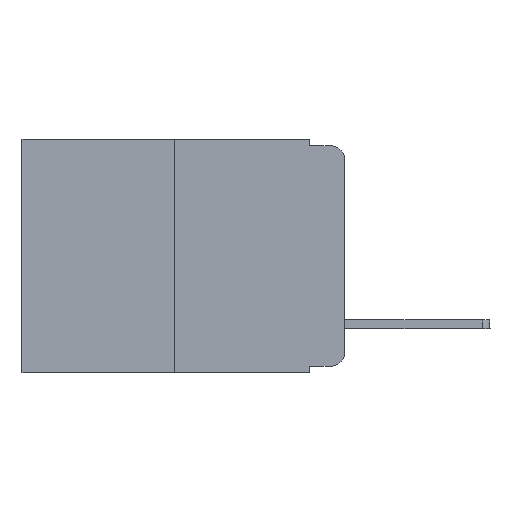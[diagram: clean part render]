
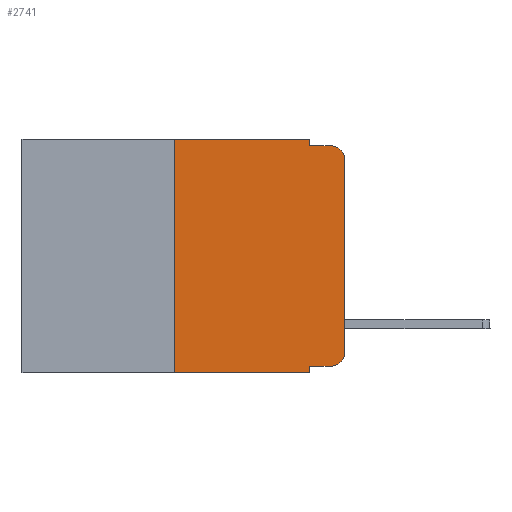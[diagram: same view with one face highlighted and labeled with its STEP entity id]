
A CAD part, left-side view. The second image highlights one B-rep face of the part: STEP entity #2741.
In plain terms, the highlighted planar face has unit normal (-1, 0, 0).
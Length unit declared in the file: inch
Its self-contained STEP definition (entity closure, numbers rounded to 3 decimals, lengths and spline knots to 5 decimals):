
#124 = VECTOR ( 'NONE', #4644, 39.37008 ) ;
#211 = EDGE_CURVE ( 'NONE', #13435, #8046, #12303, .T. ) ;
#518 = EDGE_CURVE ( 'NONE', #3727, #5119, #7516, .T. ) ;
#966 = ORIENTED_EDGE ( 'NONE', *, *, #2145, .T. ) ;
#1111 = VECTOR ( 'NONE', #12831, 39.37008 ) ;
#1455 = VERTEX_POINT ( 'NONE', #7439 ) ;
#1536 = CARTESIAN_POINT ( 'NONE',  ( 0., 0.473, 0. ) ) ;
#1609 = ORIENTED_EDGE ( 'NONE', *, *, #13899, .T. ) ;
#1706 = LINE ( 'NONE', #11536, #1111 ) ;
#1962 = CARTESIAN_POINT ( 'NONE',  ( 0., 0.25, -0.343 ) ) ;
#2133 = CARTESIAN_POINT ( 'NONE',  ( 0., 0.02, -0.01 ) ) ;
#2145 = EDGE_CURVE ( 'NONE', #16612, #15580, #2423, .T. ) ;
#2423 = LINE ( 'NONE', #12483, #6634 ) ;
#2518 = AXIS2_PLACEMENT_3D ( 'NONE', #11766, #15399, #14137 ) ;
#2538 = EDGE_CURVE ( 'NONE', #15580, #13642, #10623, .T. ) ;
#2741 = ADVANCED_FACE ( 'NONE', ( #5210 ), #16152, .F. ) ;
#3237 = DIRECTION ( 'NONE',  ( -1., 0., 0. ) ) ;
#3691 = CARTESIAN_POINT ( 'NONE',  ( 0., 0.051, 0. ) ) ;
#3693 = DIRECTION ( 'NONE',  ( 0., 0., -1. ) ) ;
#3702 = VECTOR ( 'NONE', #6491, 39.37008 ) ;
#3727 = VERTEX_POINT ( 'NONE', #7046 ) ;
#4431 = ORIENTED_EDGE ( 'NONE', *, *, #518, .F. ) ;
#4644 = DIRECTION ( 'NONE',  ( 0., -1., 0. ) ) ;
#4692 = VECTOR ( 'NONE', #10148, 39.37008 ) ;
#5088 = EDGE_CURVE ( 'NONE', #13435, #1455, #7378, .T. ) ;
#5119 = VERTEX_POINT ( 'NONE', #8451 ) ;
#5207 = CARTESIAN_POINT ( 'NONE',  ( 0., 0.051, -0.333 ) ) ;
#5210 = FACE_OUTER_BOUND ( 'NONE', #14205, .T. ) ;
#5628 = CARTESIAN_POINT ( 'NONE',  ( 0., 0.25, 0. ) ) ;
#5692 = LINE ( 'NONE', #1536, #3702 ) ;
#5862 = LINE ( 'NONE', #7553, #15664 ) ;
#6204 = DIRECTION ( 'NONE',  ( 1., 0., 0. ) ) ;
#6212 = ORIENTED_EDGE ( 'NONE', *, *, #6629, .T. ) ;
#6491 = DIRECTION ( 'NONE',  ( 0., -1., 0. ) ) ;
#6629 = EDGE_CURVE ( 'NONE', #8428, #8046, #1706, .T. ) ;
#6634 = VECTOR ( 'NONE', #13906, 39.37008 ) ;
#6912 = ORIENTED_EDGE ( 'NONE', *, *, #8570, .F. ) ;
#7046 = CARTESIAN_POINT ( 'NONE',  ( 0., 0.051, 0. ) ) ;
#7064 = ORIENTED_EDGE ( 'NONE', *, *, #5088, .T. ) ;
#7378 = LINE ( 'NONE', #12021, #124 ) ;
#7439 = CARTESIAN_POINT ( 'NONE',  ( 0., 0.02, -0.333 ) ) ;
#7502 = DIRECTION ( 'NONE',  ( 0., 0., -1. ) ) ;
#7516 = LINE ( 'NONE', #12786, #4692 ) ;
#7553 = CARTESIAN_POINT ( 'NONE',  ( 0., 0.25, 0. ) ) ;
#7783 = AXIS2_PLACEMENT_3D ( 'NONE', #16613, #6204, #3693 ) ;
#8046 = VERTEX_POINT ( 'NONE', #16294 ) ;
#8428 = VERTEX_POINT ( 'NONE', #1962 ) ;
#8451 = CARTESIAN_POINT ( 'NONE',  ( 0., 0.051, -0.01 ) ) ;
#8570 = EDGE_CURVE ( 'NONE', #8428, #11552, #5862, .T. ) ;
#8942 = AXIS2_PLACEMENT_3D ( 'NONE', #10906, #3237, #10852 ) ;
#9496 = CIRCLE ( 'NONE', #2518, 0.02 ) ;
#9533 = CARTESIAN_POINT ( 'NONE',  ( 0., 0., -0.313 ) ) ;
#10119 = VECTOR ( 'NONE', #7502, 39.37008 ) ;
#10148 = DIRECTION ( 'NONE',  ( 0., 0., -1. ) ) ;
#10186 = ORIENTED_EDGE ( 'NONE', *, *, #211, .F. ) ;
#10623 = CIRCLE ( 'NONE', #8942, 0.02 ) ;
#10852 = DIRECTION ( 'NONE',  ( 0., 0., -1. ) ) ;
#10906 = CARTESIAN_POINT ( 'NONE',  ( 0., 0.02, -0.03 ) ) ;
#11024 = DIRECTION ( 'NONE',  ( 0., -1., 0. ) ) ;
#11105 = LINE ( 'NONE', #13787, #12522 ) ;
#11536 = CARTESIAN_POINT ( 'NONE',  ( 0., 0.473, -0.343 ) ) ;
#11552 = VERTEX_POINT ( 'NONE', #5628 ) ;
#11766 = CARTESIAN_POINT ( 'NONE',  ( 0., 0.02, -0.313 ) ) ;
#12021 = CARTESIAN_POINT ( 'NONE',  ( 0., 0.051, -0.333 ) ) ;
#12303 = LINE ( 'NONE', #3691, #10119 ) ;
#12323 = CARTESIAN_POINT ( 'NONE',  ( 0., 0., -0.03 ) ) ;
#12483 = CARTESIAN_POINT ( 'NONE',  ( 0., 0., 0. ) ) ;
#12522 = VECTOR ( 'NONE', #11024, 39.37008 ) ;
#12608 = ORIENTED_EDGE ( 'NONE', *, *, #2538, .T. ) ;
#12634 = ORIENTED_EDGE ( 'NONE', *, *, #13491, .F. ) ;
#12786 = CARTESIAN_POINT ( 'NONE',  ( 0., 0.051, 0. ) ) ;
#12831 = DIRECTION ( 'NONE',  ( 0., -1., 0. ) ) ;
#13192 = EDGE_CURVE ( 'NONE', #5119, #13642, #11105, .T. ) ;
#13435 = VERTEX_POINT ( 'NONE', #5207 ) ;
#13491 = EDGE_CURVE ( 'NONE', #11552, #3727, #5692, .T. ) ;
#13642 = VERTEX_POINT ( 'NONE', #2133 ) ;
#13787 = CARTESIAN_POINT ( 'NONE',  ( 0., 0.051, -0.01 ) ) ;
#13894 = ORIENTED_EDGE ( 'NONE', *, *, #13192, .F. ) ;
#13899 = EDGE_CURVE ( 'NONE', #1455, #16612, #9496, .T. ) ;
#13906 = DIRECTION ( 'NONE',  ( 0., 0., 1. ) ) ;
#14137 = DIRECTION ( 'NONE',  ( 0., 0., -1. ) ) ;
#14205 = EDGE_LOOP ( 'NONE', ( #966, #12608, #13894, #4431, #12634, #6912, #6212, #10186, #7064, #1609 ) ) ;
#15373 = DIRECTION ( 'NONE',  ( 0., 0., 1. ) ) ;
#15399 = DIRECTION ( 'NONE',  ( -1., 0., 0. ) ) ;
#15580 = VERTEX_POINT ( 'NONE', #12323 ) ;
#15664 = VECTOR ( 'NONE', #15373, 39.37008 ) ;
#16152 = PLANE ( 'NONE',  #7783 ) ;
#16294 = CARTESIAN_POINT ( 'NONE',  ( 0., 0.051, -0.343 ) ) ;
#16612 = VERTEX_POINT ( 'NONE', #9533 ) ;
#16613 = CARTESIAN_POINT ( 'NONE',  ( 0., 0.473, 0. ) ) ;
